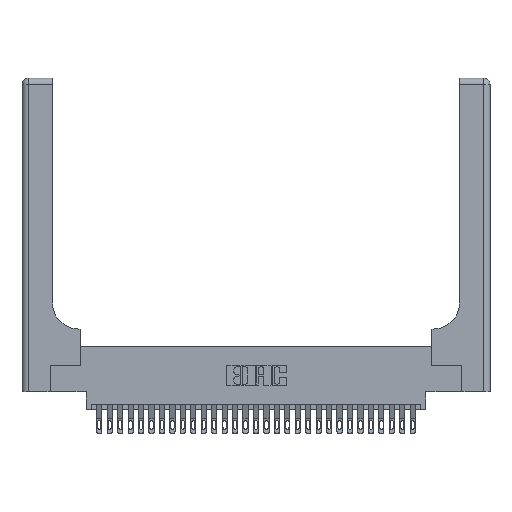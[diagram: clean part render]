
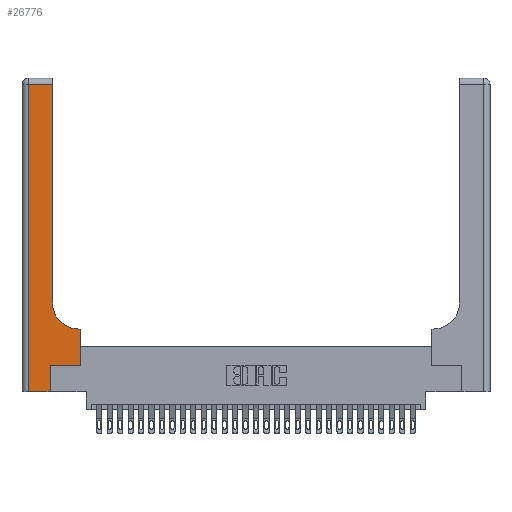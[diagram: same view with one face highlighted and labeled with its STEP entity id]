
A CAD part, top view. The second image highlights one B-rep face of the part: STEP entity #26776.
In plain terms, the highlighted planar face has unit normal (0, 0, 1).
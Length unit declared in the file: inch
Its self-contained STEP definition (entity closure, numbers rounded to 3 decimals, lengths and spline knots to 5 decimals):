
#667 = CARTESIAN_POINT ( 'NONE',  ( 0.06, 0., 0.37 ) ) ;
#762 = VECTOR ( 'NONE', #24782, 39.37008 ) ;
#1512 = AXIS2_PLACEMENT_3D ( 'NONE', #6417, #8866, #25877 ) ;
#1570 = LINE ( 'NONE', #19901, #762 ) ;
#2158 = VERTEX_POINT ( 'NONE', #23809 ) ;
#2720 = LINE ( 'NONE', #15542, #27848 ) ;
#3187 = CARTESIAN_POINT ( 'NONE',  ( 0.5585, 0.6, 0.37 ) ) ;
#3784 = EDGE_CURVE ( 'NONE', #25930, #25662, #10542, .T. ) ;
#4200 = EDGE_CURVE ( 'NONE', #10738, #2158, #31347, .T. ) ;
#4501 = DIRECTION ( 'NONE',  ( 1., 0., 0. ) ) ;
#4648 = ORIENTED_EDGE ( 'NONE', *, *, #3784, .T. ) ;
#4694 = CARTESIAN_POINT ( 'NONE',  ( 0.269, 0.25, 0.37 ) ) ;
#5008 = ORIENTED_EDGE ( 'NONE', *, *, #9372, .T. ) ;
#5411 = CIRCLE ( 'NONE', #23385, 0.25 ) ;
#5662 = LINE ( 'NONE', #23115, #24348 ) ;
#6344 = CARTESIAN_POINT ( 'NONE',  ( 0., 2.94, 0.37 ) ) ;
#6417 = CARTESIAN_POINT ( 'NONE',  ( 0., 3., 0.37 ) ) ;
#6546 = EDGE_CURVE ( 'NONE', #24699, #22721, #5411, .T. ) ;
#7895 = EDGE_CURVE ( 'NONE', #22721, #10738, #1570, .T. ) ;
#8866 = DIRECTION ( 'NONE',  ( 0., 0., -1. ) ) ;
#9372 = EDGE_CURVE ( 'NONE', #25662, #29654, #5662, .T. ) ;
#9412 = VECTOR ( 'NONE', #28667, 39.37008 ) ;
#9712 = LINE ( 'NONE', #16723, #28341 ) ;
#9915 = EDGE_CURVE ( 'NONE', #29654, #21436, #9712, .T. ) ;
#10069 = FACE_OUTER_BOUND ( 'NONE', #10873, .T. ) ;
#10542 = LINE ( 'NONE', #26756, #17099 ) ;
#10659 = DIRECTION ( 'NONE',  ( 0., -1., 0. ) ) ;
#10738 = VERTEX_POINT ( 'NONE', #22153 ) ;
#10873 = EDGE_LOOP ( 'NONE', ( #20508, #29892, #20366, #4648, #5008, #22824, #24050, #18728, #15351 ) ) ;
#10982 = DIRECTION ( 'NONE',  ( 0., 1., 0. ) ) ;
#12259 = DIRECTION ( 'NONE',  ( 1., 0., 0. ) ) ;
#12655 = CARTESIAN_POINT ( 'NONE',  ( 0.5415, 0.85, 0.37 ) ) ;
#15113 = DIRECTION ( 'NONE',  ( 1., 0., 0. ) ) ;
#15351 = ORIENTED_EDGE ( 'NONE', *, *, #6546, .T. ) ;
#15542 = CARTESIAN_POINT ( 'NONE',  ( 0.5585, 0.25, 0.37 ) ) ;
#16723 = CARTESIAN_POINT ( 'NONE',  ( 0.269, 0.25, 0.37 ) ) ;
#17099 = VECTOR ( 'NONE', #12259, 39.37008 ) ;
#17268 = CARTESIAN_POINT ( 'NONE',  ( 0.2915, 0.85, 0.37 ) ) ;
#17388 = EDGE_CURVE ( 'NONE', #2158, #25930, #27652, .T. ) ;
#18728 = ORIENTED_EDGE ( 'NONE', *, *, #31465, .T. ) ;
#19724 = VECTOR ( 'NONE', #10659, 39.37008 ) ;
#19901 = CARTESIAN_POINT ( 'NONE',  ( 0.2915, 3., 0.37 ) ) ;
#20366 = ORIENTED_EDGE ( 'NONE', *, *, #17388, .T. ) ;
#20508 = ORIENTED_EDGE ( 'NONE', *, *, #7895, .T. ) ;
#20846 = VECTOR ( 'NONE', #23393, 39.37008 ) ;
#20973 = EDGE_CURVE ( 'NONE', #21436, #26566, #2720, .T. ) ;
#21019 = PLANE ( 'NONE',  #1512 ) ;
#21436 = VERTEX_POINT ( 'NONE', #27110 ) ;
#22153 = CARTESIAN_POINT ( 'NONE',  ( 0.2915, 2.94, 0.37 ) ) ;
#22721 = VERTEX_POINT ( 'NONE', #17268 ) ;
#22824 = ORIENTED_EDGE ( 'NONE', *, *, #9915, .T. ) ;
#22832 = DIRECTION ( 'NONE',  ( 0., 1., 0. ) ) ;
#23115 = CARTESIAN_POINT ( 'NONE',  ( 0.269, 0., 0.37 ) ) ;
#23385 = AXIS2_PLACEMENT_3D ( 'NONE', #12655, #29555, #15113 ) ;
#23393 = DIRECTION ( 'NONE',  ( -1., 0., 0. ) ) ;
#23657 = CARTESIAN_POINT ( 'NONE',  ( 0.269, 0., 0.37 ) ) ;
#23809 = CARTESIAN_POINT ( 'NONE',  ( 0.06, 2.94, 0.37 ) ) ;
#23855 = CARTESIAN_POINT ( 'NONE',  ( 0.2915, 0.6, 0.37 ) ) ;
#24050 = ORIENTED_EDGE ( 'NONE', *, *, #20973, .T. ) ;
#24348 = VECTOR ( 'NONE', #10982, 39.37008 ) ;
#24699 = VERTEX_POINT ( 'NONE', #26836 ) ;
#24782 = DIRECTION ( 'NONE',  ( 0., 1., 0. ) ) ;
#25662 = VERTEX_POINT ( 'NONE', #23657 ) ;
#25877 = DIRECTION ( 'NONE',  ( -1., 0., 0. ) ) ;
#25930 = VERTEX_POINT ( 'NONE', #667 ) ;
#26566 = VERTEX_POINT ( 'NONE', #3187 ) ;
#26756 = CARTESIAN_POINT ( 'NONE',  ( 0., 0., 0.37 ) ) ;
#26776 = ADVANCED_FACE ( 'NONE', ( #10069 ), #21019, .F. ) ;
#26836 = CARTESIAN_POINT ( 'NONE',  ( 0.5415, 0.6, 0.37 ) ) ;
#27110 = CARTESIAN_POINT ( 'NONE',  ( 0.5585, 0.25, 0.37 ) ) ;
#27652 = LINE ( 'NONE', #30050, #19724 ) ;
#27848 = VECTOR ( 'NONE', #22832, 39.37008 ) ;
#28341 = VECTOR ( 'NONE', #4501, 39.37008 ) ;
#28667 = DIRECTION ( 'NONE',  ( -1., 0., 0. ) ) ;
#29514 = LINE ( 'NONE', #23855, #9412 ) ;
#29555 = DIRECTION ( 'NONE',  ( 0., 0., -1. ) ) ;
#29654 = VERTEX_POINT ( 'NONE', #4694 ) ;
#29892 = ORIENTED_EDGE ( 'NONE', *, *, #4200, .T. ) ;
#30050 = CARTESIAN_POINT ( 'NONE',  ( 0.06, 3., 0.37 ) ) ;
#31347 = LINE ( 'NONE', #6344, #20846 ) ;
#31465 = EDGE_CURVE ( 'NONE', #26566, #24699, #29514, .T. ) ;
